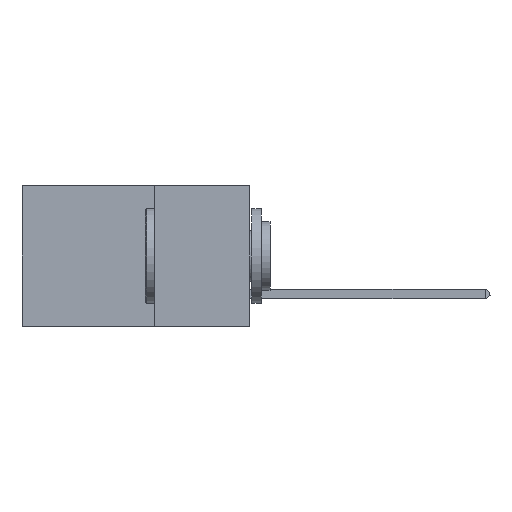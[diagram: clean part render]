
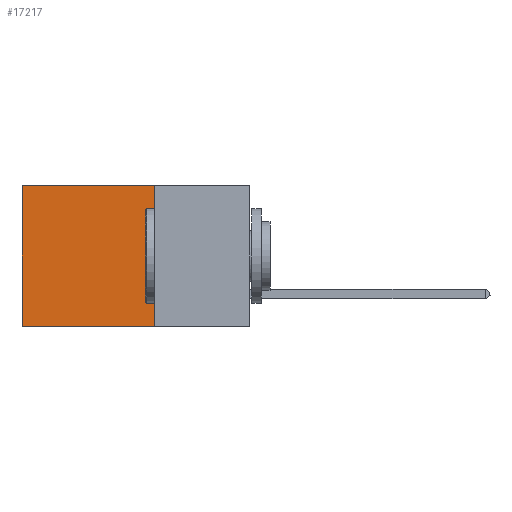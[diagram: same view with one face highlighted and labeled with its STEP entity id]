
A CAD part, left-side view. The second image highlights one B-rep face of the part: STEP entity #17217.
In plain terms, the highlighted planar face has unit normal (-1, 0, 0).
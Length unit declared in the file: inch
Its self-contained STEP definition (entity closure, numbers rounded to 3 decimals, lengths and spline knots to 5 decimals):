
#174 = EDGE_CURVE ( 'NONE', #6174, #24151, #18851, .T. ) ;
#908 = LINE ( 'NONE', #18119, #7623 ) ;
#1258 = VERTEX_POINT ( 'NONE', #13679 ) ;
#1432 = AXIS2_PLACEMENT_3D ( 'NONE', #30544, #12185, #30899 ) ;
#2074 = DIRECTION ( 'NONE',  ( 0., 1., 0. ) ) ;
#3018 = ORIENTED_EDGE ( 'NONE', *, *, #5960, .T. ) ;
#4412 = VECTOR ( 'NONE', #5955, 39.37008 ) ;
#4960 = EDGE_LOOP ( 'NONE', ( #3018, #18385, #34120, #27075 ) ) ;
#5309 = FACE_OUTER_BOUND ( 'NONE', #4960, .T. ) ;
#5955 = DIRECTION ( 'NONE',  ( 0., 1., 0. ) ) ;
#5960 = EDGE_CURVE ( 'NONE', #1258, #14697, #7650, .T. ) ;
#6174 = VERTEX_POINT ( 'NONE', #20151 ) ;
#6200 = CARTESIAN_POINT ( 'NONE',  ( 0.2875, 0.25, -0.37 ) ) ;
#6265 = VECTOR ( 'NONE', #33903, 39.37008 ) ;
#7623 = VECTOR ( 'NONE', #2074, 39.37008 ) ;
#7650 = LINE ( 'NONE', #29161, #10616 ) ;
#10480 = EDGE_CURVE ( 'NONE', #24151, #14697, #32501, .T. ) ;
#10616 = VECTOR ( 'NONE', #32076, 39.37008 ) ;
#12185 = DIRECTION ( 'NONE',  ( 1., 0., 0. ) ) ;
#13679 = CARTESIAN_POINT ( 'NONE',  ( 0.2875, 0.6, 0. ) ) ;
#13991 = EDGE_CURVE ( 'NONE', #6174, #1258, #908, .T. ) ;
#14697 = VERTEX_POINT ( 'NONE', #27401 ) ;
#17217 = ADVANCED_FACE ( 'NONE', ( #5309 ), #25628, .F. ) ;
#18119 = CARTESIAN_POINT ( 'NONE',  ( 0.2875, 0.25, 0. ) ) ;
#18385 = ORIENTED_EDGE ( 'NONE', *, *, #10480, .F. ) ;
#18851 = LINE ( 'NONE', #25459, #6265 ) ;
#20151 = CARTESIAN_POINT ( 'NONE',  ( 0.2875, 0.25, 0. ) ) ;
#23519 = CARTESIAN_POINT ( 'NONE',  ( 0.2875, 0.25, -0.37 ) ) ;
#24151 = VERTEX_POINT ( 'NONE', #23519 ) ;
#25459 = CARTESIAN_POINT ( 'NONE',  ( 0.2875, 0.25, 0. ) ) ;
#25628 = PLANE ( 'NONE',  #1432 ) ;
#27075 = ORIENTED_EDGE ( 'NONE', *, *, #13991, .T. ) ;
#27401 = CARTESIAN_POINT ( 'NONE',  ( 0.2875, 0.6, -0.37 ) ) ;
#29161 = CARTESIAN_POINT ( 'NONE',  ( 0.2875, 0.6, 0. ) ) ;
#30544 = CARTESIAN_POINT ( 'NONE',  ( 0.2875, 0.25, 0. ) ) ;
#30899 = DIRECTION ( 'NONE',  ( 0., 0., -1. ) ) ;
#32076 = DIRECTION ( 'NONE',  ( 0., 0., -1. ) ) ;
#32501 = LINE ( 'NONE', #6200, #4412 ) ;
#33903 = DIRECTION ( 'NONE',  ( 0., 0., -1. ) ) ;
#34120 = ORIENTED_EDGE ( 'NONE', *, *, #174, .F. ) ;
